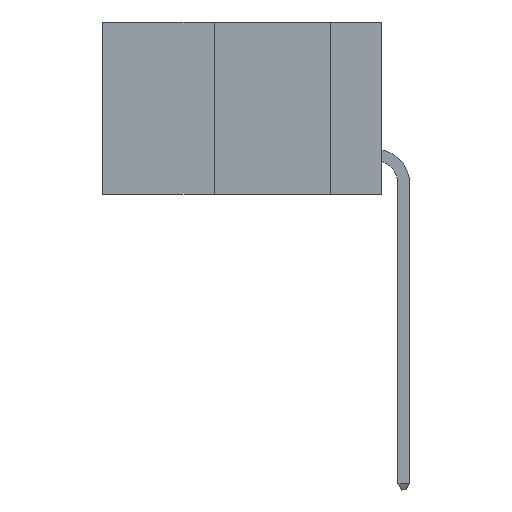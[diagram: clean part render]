
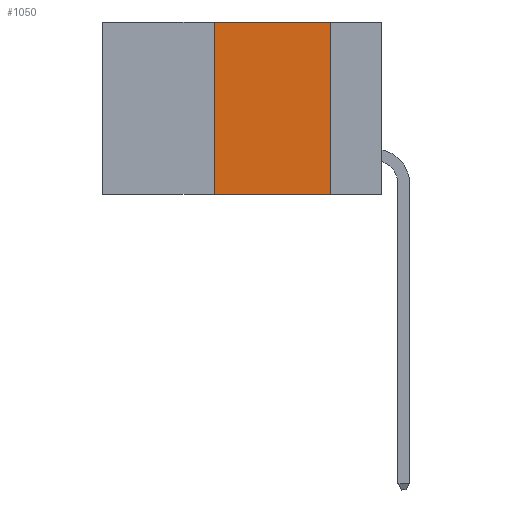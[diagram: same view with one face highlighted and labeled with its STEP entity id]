
A CAD part, left-side view. The second image highlights one B-rep face of the part: STEP entity #1050.
In plain terms, the highlighted planar face has unit normal (-1, 0, 0).
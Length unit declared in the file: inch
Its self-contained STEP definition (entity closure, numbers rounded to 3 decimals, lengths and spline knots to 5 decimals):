
#107 = VERTEX_POINT ( 'NONE', #14558 ) ;
#536 = CARTESIAN_POINT ( 'NONE',  ( 0., 0.11, 0. ) ) ;
#1050 = ADVANCED_FACE ( 'NONE', ( #3907 ), #10729, .F. ) ;
#1135 = DIRECTION ( 'NONE',  ( 0., -1., 0. ) ) ;
#1327 = ORIENTED_EDGE ( 'NONE', *, *, #9037, .F. ) ;
#1361 = EDGE_CURVE ( 'NONE', #10438, #107, #2061, .T. ) ;
#1956 = DIRECTION ( 'NONE',  ( 0., -1., 0. ) ) ;
#2061 = LINE ( 'NONE', #7627, #8990 ) ;
#2959 = CARTESIAN_POINT ( 'NONE',  ( 0., 0.6, 0. ) ) ;
#3116 = ORIENTED_EDGE ( 'NONE', *, *, #3512, .F. ) ;
#3259 = ORIENTED_EDGE ( 'NONE', *, *, #5467, .F. ) ;
#3512 = EDGE_CURVE ( 'NONE', #10438, #10363, #5623, .T. ) ;
#3555 = DIRECTION ( 'NONE',  ( 0., 0., 1. ) ) ;
#3656 = CARTESIAN_POINT ( 'NONE',  ( 0., 0.36, -0.37 ) ) ;
#3907 = FACE_OUTER_BOUND ( 'NONE', #5347, .T. ) ;
#4059 = ORIENTED_EDGE ( 'NONE', *, *, #1361, .T. ) ;
#4240 = DIRECTION ( 'NONE',  ( 1., 0., 0. ) ) ;
#5347 = EDGE_LOOP ( 'NONE', ( #3259, #1327, #3116, #4059 ) ) ;
#5467 = EDGE_CURVE ( 'NONE', #9595, #107, #15037, .T. ) ;
#5583 = CARTESIAN_POINT ( 'NONE',  ( 0., 0.6, 0. ) ) ;
#5623 = LINE ( 'NONE', #11283, #8676 ) ;
#6982 = LINE ( 'NONE', #5583, #10023 ) ;
#7627 = CARTESIAN_POINT ( 'NONE',  ( 0., 0.6, -0.37 ) ) ;
#8676 = VECTOR ( 'NONE', #3555, 39.37008 ) ;
#8990 = VECTOR ( 'NONE', #1135, 39.37008 ) ;
#9037 = EDGE_CURVE ( 'NONE', #10363, #9595, #6982, .T. ) ;
#9243 = AXIS2_PLACEMENT_3D ( 'NONE', #2959, #4240, #15961 ) ;
#9515 = DIRECTION ( 'NONE',  ( 0., 0., -1. ) ) ;
#9595 = VERTEX_POINT ( 'NONE', #16080 ) ;
#10023 = VECTOR ( 'NONE', #1956, 39.37008 ) ;
#10363 = VERTEX_POINT ( 'NONE', #16893 ) ;
#10438 = VERTEX_POINT ( 'NONE', #3656 ) ;
#10729 = PLANE ( 'NONE',  #9243 ) ;
#11283 = CARTESIAN_POINT ( 'NONE',  ( 0., 0.36, 0. ) ) ;
#13569 = VECTOR ( 'NONE', #9515, 39.37008 ) ;
#14558 = CARTESIAN_POINT ( 'NONE',  ( 0., 0.11, -0.37 ) ) ;
#15037 = LINE ( 'NONE', #536, #13569 ) ;
#15961 = DIRECTION ( 'NONE',  ( 0., 0., -1. ) ) ;
#16080 = CARTESIAN_POINT ( 'NONE',  ( 0., 0.11, 0. ) ) ;
#16893 = CARTESIAN_POINT ( 'NONE',  ( 0., 0.36, 0. ) ) ;
